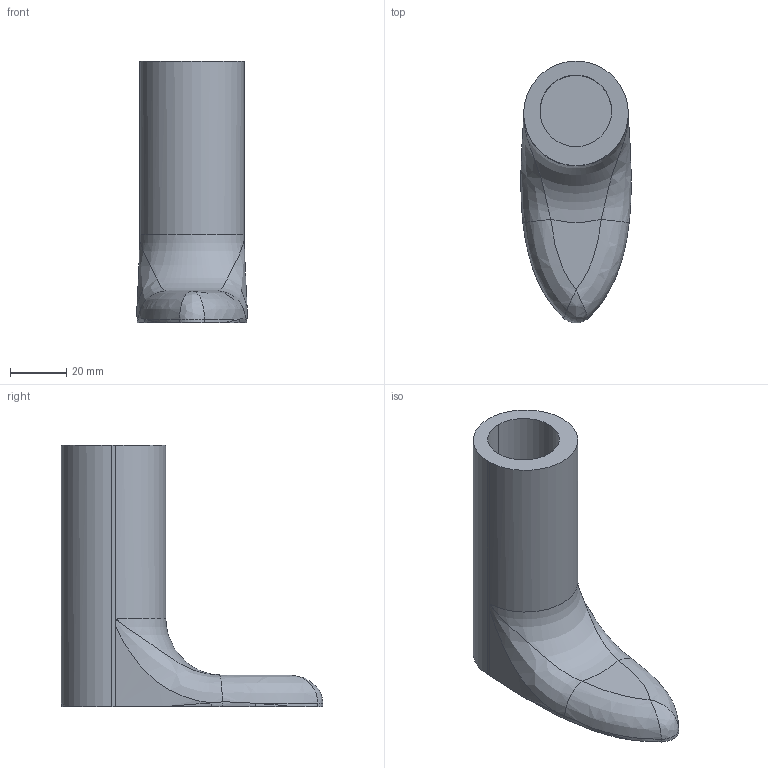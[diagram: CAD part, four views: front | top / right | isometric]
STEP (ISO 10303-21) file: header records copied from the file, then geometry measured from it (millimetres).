
FILE_DESCRIPTION (( 'STEP AP214' ), '1' );
FILE_NAME ('8.STEP', '2013-09-29T07:08:00', ( 'elpi' ), ( '' ), 'SwSTEP 2.0', 'SolidWorks 2013', '' );
FILE_SCHEMA (( 'AUTOMOTIVE_DESIGN' ));
Length unit declared in the file: millimetre
Products named in the file (1): 8
Bounding box: 39.17 x 92.86 x 92.8 mm (x, y, z)
Volume: 82142.4 mm3; surface area: 23789.9 mm2
Topology: 1 solids, 1 shells, 30 faces, 69 edges, 41 vertices
Faces by surface type: bspline 18, plane 6, cylinder 5, torus 1
Entity records: 1746 total; most frequent: CARTESIAN_POINT 1160, ORIENTED_EDGE 136, DIRECTION 80, EDGE_CURVE 68, VERTEX_POINT 41, B_SPLINE_CURVE_WITH_KNOTS 34, AXIS2_PLACEMENT_3D 33, EDGE_LOOP 31
